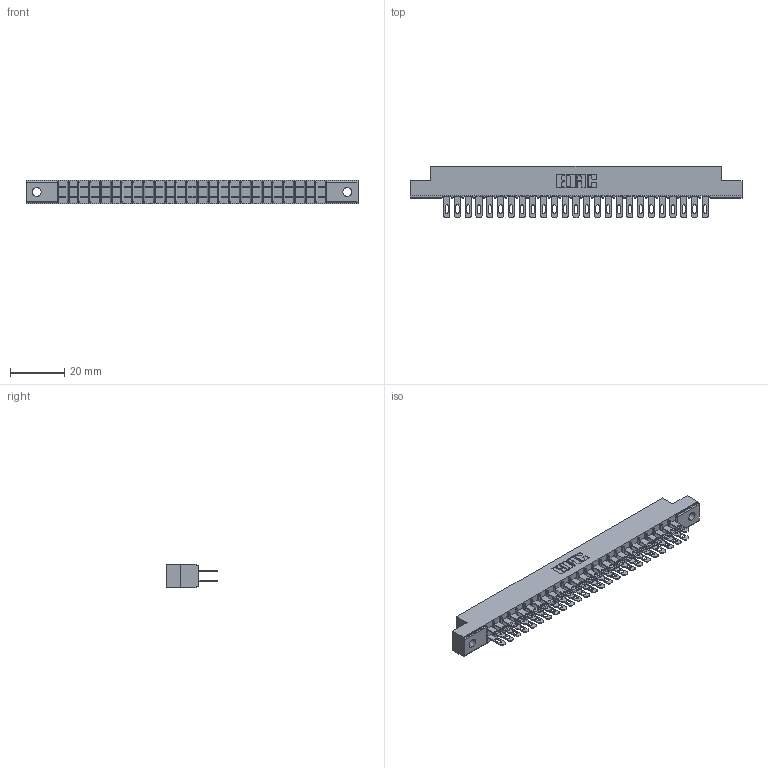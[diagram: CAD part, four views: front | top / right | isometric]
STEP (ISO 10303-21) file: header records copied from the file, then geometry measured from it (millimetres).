
FILE_DESCRIPTION (( 'STEP AP203' ), '1' );
FILE_NAME ('305-050-500-502.STEP', '2019-09-09T21:32:11', ( '' ), ( '' ), 'SwSTEP 2.0', 'SolidWorks 2016', '' );
FILE_SCHEMA (( 'CONFIG_CONTROL_DESIGN' ));
Length unit declared in the file: inch
Products named in the file (3): 305 Part_.128 Dia; 305-050-500-502; 305-290-001_500
Assembly tree (51 placements, depth 2):
  305-050-500-502
    305 Part_.128 Dia
    305-290-001_500  x50
Bounding box: 122.07 x 18.85 x 8.71 mm (x, y, z)
Volume: 7421 mm3; surface area: 15595.5 mm2
Topology: 51 solids, 51 shells, 2616 faces, 7491 edges, 4858 vertices
Faces by surface type: plane 1468, cylinder 1048, sphere 100
Entity records: 29162 total; most frequent: CARTESIAN_POINT 4825, ORIENTED_EDGE 4786, DIRECTION 4683, EDGE_CURVE 2393, VECTOR 1915, LINE 1915, VERTEX_POINT 1526, AXIS2_PLACEMENT_3D 1384
